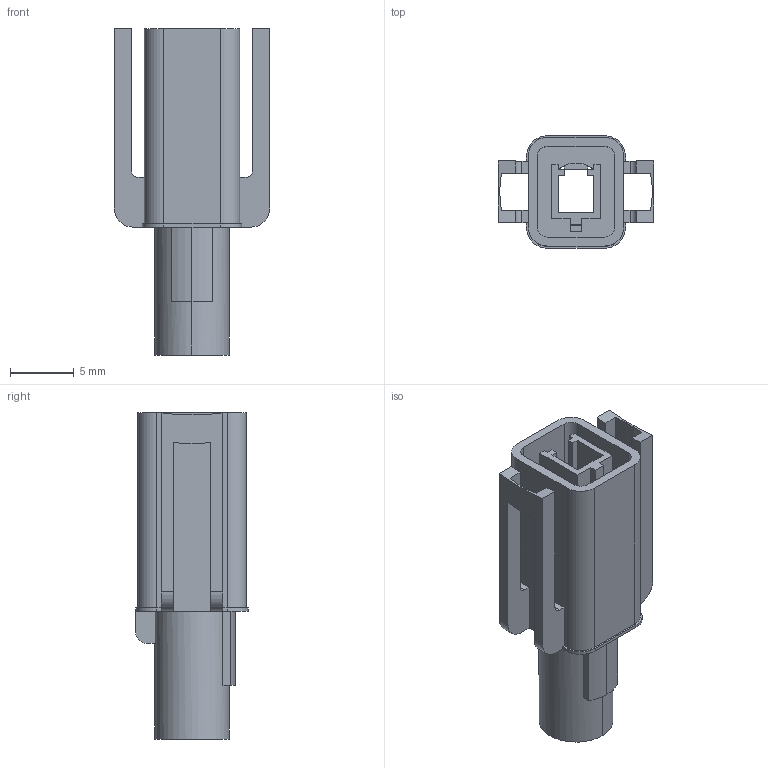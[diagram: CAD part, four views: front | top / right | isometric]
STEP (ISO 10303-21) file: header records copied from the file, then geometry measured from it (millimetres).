
FILE_DESCRIPTION (( 'STEP AP214' ), '1' );
FILE_NAME ('568-001-000-200.STEP', '2020-07-29T15:50:05', ( '' ), ( '' ), 'SwSTEP 2.0', 'SolidWorks 2020', '' );
FILE_SCHEMA (( 'AUTOMOTIVE_DESIGN' ));
Length unit declared in the file: millimetre
Products named in the file (1): 568-001-000-200
Bounding box: 12.15 x 8.8 x 25.5 mm (x, y, z)
Volume: 628.2 mm3; surface area: 2017.1 mm2
Topology: 1 solids, 1 shells, 109 faces, 328 edges, 218 vertices
Faces by surface type: plane 73, cylinder 36
Entity records: 3736 total; most frequent: CARTESIAN_POINT 678, ORIENTED_EDGE 656, DIRECTION 616, EDGE_CURVE 328, VECTOR 248, LINE 248, VERTEX_POINT 218, AXIS2_PLACEMENT_3D 184
